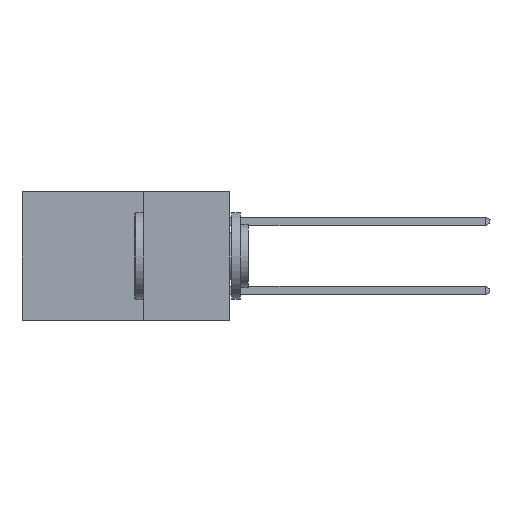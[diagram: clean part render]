
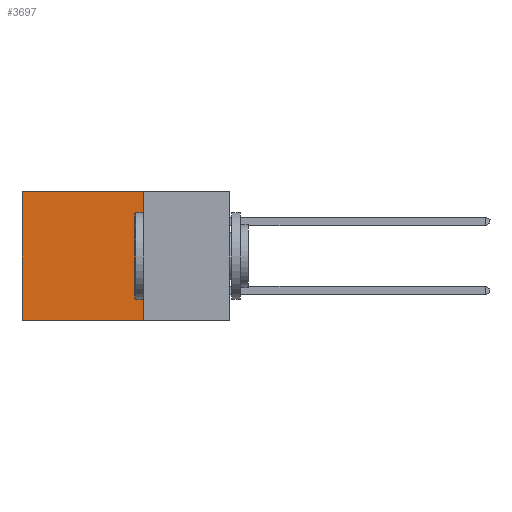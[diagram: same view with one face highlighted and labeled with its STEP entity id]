
A CAD part, left-side view. The second image highlights one B-rep face of the part: STEP entity #3697.
In plain terms, the highlighted planar face has unit normal (-1, 0, 0).
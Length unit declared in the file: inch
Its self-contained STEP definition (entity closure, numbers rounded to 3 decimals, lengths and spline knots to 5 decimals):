
#21 = ORIENTED_EDGE ( 'NONE', *, *, #6981, .F. ) ;
#118 = VERTEX_POINT ( 'NONE', #9823 ) ;
#231 = EDGE_CURVE ( 'NONE', #21135, #9848, #2857, .T. ) ;
#1932 = DIRECTION ( 'NONE',  ( 1., 0., 0. ) ) ;
#2393 = CARTESIAN_POINT ( 'NONE',  ( 0.2615, 0.25, -0.37 ) ) ;
#2857 = LINE ( 'NONE', #8053, #21375 ) ;
#3697 = ADVANCED_FACE ( 'NONE', ( #10330 ), #20402, .F. ) ;
#3733 = DIRECTION ( 'NONE',  ( 0., 1., 0. ) ) ;
#3832 = CARTESIAN_POINT ( 'NONE',  ( 0.2615, 0.25, -0.37 ) ) ;
#4450 = ORIENTED_EDGE ( 'NONE', *, *, #231, .T. ) ;
#5661 = DIRECTION ( 'NONE',  ( 0., 1., 0. ) ) ;
#6390 = EDGE_LOOP ( 'NONE', ( #4450, #21, #17013, #18714 ) ) ;
#6981 = EDGE_CURVE ( 'NONE', #16715, #9848, #12358, .T. ) ;
#7094 = EDGE_CURVE ( 'NONE', #118, #16715, #17556, .T. ) ;
#7252 = CARTESIAN_POINT ( 'NONE',  ( 0.2615, 0.6, -0.37 ) ) ;
#8053 = CARTESIAN_POINT ( 'NONE',  ( 0.2615, 0.6, -0.37 ) ) ;
#8675 = DIRECTION ( 'NONE',  ( 0., 0., -1. ) ) ;
#9136 = DIRECTION ( 'NONE',  ( 0., 0., -1. ) ) ;
#9171 = EDGE_CURVE ( 'NONE', #118, #21135, #15723, .T. ) ;
#9823 = CARTESIAN_POINT ( 'NONE',  ( 0.2615, 0.25, 0. ) ) ;
#9848 = VERTEX_POINT ( 'NONE', #7252 ) ;
#10330 = FACE_OUTER_BOUND ( 'NONE', #6390, .T. ) ;
#11265 = DIRECTION ( 'NONE',  ( 0., 0., -1. ) ) ;
#12358 = LINE ( 'NONE', #18990, #18120 ) ;
#15723 = LINE ( 'NONE', #15831, #19944 ) ;
#15831 = CARTESIAN_POINT ( 'NONE',  ( 0.2615, 0.25, 0. ) ) ;
#16019 = VECTOR ( 'NONE', #9136, 39.37008 ) ;
#16715 = VERTEX_POINT ( 'NONE', #3832 ) ;
#17013 = ORIENTED_EDGE ( 'NONE', *, *, #7094, .F. ) ;
#17556 = LINE ( 'NONE', #2393, #16019 ) ;
#18120 = VECTOR ( 'NONE', #3733, 39.37008 ) ;
#18714 = ORIENTED_EDGE ( 'NONE', *, *, #9171, .T. ) ;
#18990 = CARTESIAN_POINT ( 'NONE',  ( 0.2615, 0.25, -0.37 ) ) ;
#19754 = CARTESIAN_POINT ( 'NONE',  ( 0.2615, 0.6, 0. ) ) ;
#19944 = VECTOR ( 'NONE', #5661, 39.37008 ) ;
#20402 = PLANE ( 'NONE',  #20559 ) ;
#20559 = AXIS2_PLACEMENT_3D ( 'NONE', #20631, #1932, #8675 ) ;
#20631 = CARTESIAN_POINT ( 'NONE',  ( 0.2615, 0.25, -0.37 ) ) ;
#21135 = VERTEX_POINT ( 'NONE', #19754 ) ;
#21375 = VECTOR ( 'NONE', #11265, 39.37008 ) ;
